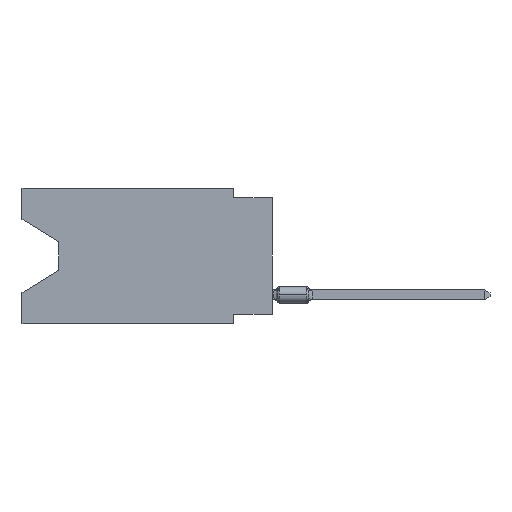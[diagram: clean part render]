
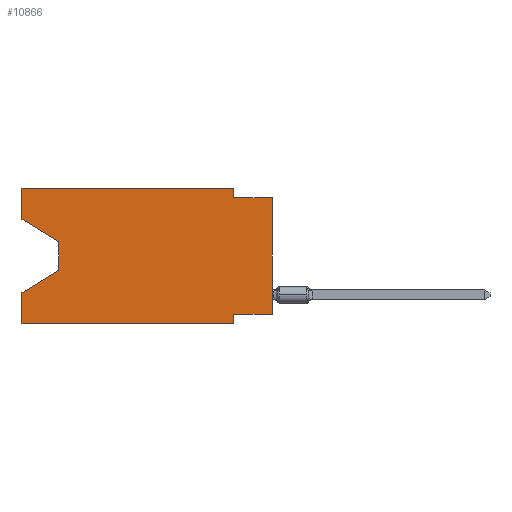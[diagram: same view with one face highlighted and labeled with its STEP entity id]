
A CAD part, left-side view. The second image highlights one B-rep face of the part: STEP entity #10866.
In plain terms, the highlighted planar face has unit normal (-1, 0, 0).
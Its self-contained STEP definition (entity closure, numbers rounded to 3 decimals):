
#94 = CARTESIAN_POINT ( 'NONE',  ( 0., 16.383, -2.038 ) ) ;
#161 = CARTESIAN_POINT ( 'NONE',  ( 0., 16.383, -6.852 ) ) ;
#174 = EDGE_CURVE ( 'NONE', #10808, #25910, #8458, .T. ) ;
#199 = CARTESIAN_POINT ( 'NONE',  ( 0., 16.383, 0. ) ) ;
#316 = DIRECTION ( 'NONE',  ( 0., 0., 1. ) ) ;
#1259 = ORIENTED_EDGE ( 'NONE', *, *, #18233, .T. ) ;
#1653 = VERTEX_POINT ( 'NONE', #4019 ) ;
#1872 = VECTOR ( 'NONE', #27531, 1000. ) ;
#2464 = CARTESIAN_POINT ( 'NONE',  ( 0., 2.54, -8.89 ) ) ;
#2564 = LINE ( 'NONE', #18908, #8574 ) ;
#3318 = VERTEX_POINT ( 'NONE', #94 ) ;
#3517 = LINE ( 'NONE', #28658, #28366 ) ;
#3856 = VECTOR ( 'NONE', #316, 1000. ) ;
#4019 = CARTESIAN_POINT ( 'NONE',  ( 0., 0., -0.635 ) ) ;
#4027 = CARTESIAN_POINT ( 'NONE',  ( 0., 13.97, -3.505 ) ) ;
#4533 = VECTOR ( 'NONE', #28274, 1000. ) ;
#4582 = CARTESIAN_POINT ( 'NONE',  ( 0., 2.54, 0. ) ) ;
#4903 = CARTESIAN_POINT ( 'NONE',  ( 0., 16.383, -2.038 ) ) ;
#4917 = ORIENTED_EDGE ( 'NONE', *, *, #6311, .T. ) ;
#5042 = CARTESIAN_POINT ( 'NONE',  ( 0., 13.97, -3.505 ) ) ;
#5176 = CARTESIAN_POINT ( 'NONE',  ( 0., 0., 0. ) ) ;
#5180 = VECTOR ( 'NONE', #23987, 1000. ) ;
#6311 = EDGE_CURVE ( 'NONE', #16733, #1653, #12278, .T. ) ;
#6521 = EDGE_CURVE ( 'NONE', #3318, #10808, #12084, .T. ) ;
#8110 = CARTESIAN_POINT ( 'NONE',  ( 0., 16.383, -8.89 ) ) ;
#8245 = ORIENTED_EDGE ( 'NONE', *, *, #27489, .F. ) ;
#8458 = LINE ( 'NONE', #24808, #15820 ) ;
#8574 = VECTOR ( 'NONE', #14290, 1000. ) ;
#9276 = CARTESIAN_POINT ( 'NONE',  ( 0., 16.383, 0. ) ) ;
#9345 = LINE ( 'NONE', #23687, #5180 ) ;
#9678 = ORIENTED_EDGE ( 'NONE', *, *, #19891, .T. ) ;
#9737 = VECTOR ( 'NONE', #12113, 1000. ) ;
#10376 = CARTESIAN_POINT ( 'NONE',  ( 0., 2.54, -0.635 ) ) ;
#10411 = LINE ( 'NONE', #19818, #9737 ) ;
#10499 = ORIENTED_EDGE ( 'NONE', *, *, #20463, .T. ) ;
#10564 = EDGE_CURVE ( 'NONE', #14357, #25654, #2564, .T. ) ;
#10687 = ORIENTED_EDGE ( 'NONE', *, *, #10564, .F. ) ;
#10729 = VERTEX_POINT ( 'NONE', #8110 ) ;
#10808 = VERTEX_POINT ( 'NONE', #13043 ) ;
#10866 = ADVANCED_FACE ( 'NONE', ( #27672 ), #20418, .F. ) ;
#11349 = VERTEX_POINT ( 'NONE', #161 ) ;
#11855 = CARTESIAN_POINT ( 'NONE',  ( 0., 2.54, -8.255 ) ) ;
#11998 = DIRECTION ( 'NONE',  ( 0., -0.855, -0.519 ) ) ;
#12084 = LINE ( 'NONE', #199, #4533 ) ;
#12113 = DIRECTION ( 'NONE',  ( 0., 0.855, -0.519 ) ) ;
#12263 = VERTEX_POINT ( 'NONE', #20882 ) ;
#12278 = LINE ( 'NONE', #5176, #25726 ) ;
#13043 = CARTESIAN_POINT ( 'NONE',  ( 0., 16.383, 0. ) ) ;
#13318 = ORIENTED_EDGE ( 'NONE', *, *, #24671, .F. ) ;
#13507 = LINE ( 'NONE', #15665, #22128 ) ;
#13980 = EDGE_CURVE ( 'NONE', #10729, #11349, #28088, .T. ) ;
#14290 = DIRECTION ( 'NONE',  ( 0., 0., -1. ) ) ;
#14357 = VERTEX_POINT ( 'NONE', #11855 ) ;
#14587 = DIRECTION ( 'NONE',  ( 0., 0., 1. ) ) ;
#15665 = CARTESIAN_POINT ( 'NONE',  ( 0., 0., -0.635 ) ) ;
#15820 = VECTOR ( 'NONE', #18325, 1000. ) ;
#16733 = VERTEX_POINT ( 'NONE', #27047 ) ;
#18233 = EDGE_CURVE ( 'NONE', #30322, #12263, #25317, .T. ) ;
#18325 = DIRECTION ( 'NONE',  ( 0., -1., 0. ) ) ;
#18405 = EDGE_LOOP ( 'NONE', ( #9678, #1259, #10499, #20678, #25299, #10687, #13318, #4917, #8245, #21248, #18439, #27879 ) ) ;
#18439 = ORIENTED_EDGE ( 'NONE', *, *, #174, .F. ) ;
#18583 = VECTOR ( 'NONE', #11998, 1000. ) ;
#18908 = CARTESIAN_POINT ( 'NONE',  ( 0., 2.54, -8.89 ) ) ;
#19818 = CARTESIAN_POINT ( 'NONE',  ( 0., 13.97, -5.385 ) ) ;
#19891 = EDGE_CURVE ( 'NONE', #3318, #30322, #30501, .T. ) ;
#20418 = PLANE ( 'NONE',  #20900 ) ;
#20463 = EDGE_CURVE ( 'NONE', #12263, #11349, #10411, .T. ) ;
#20676 = DIRECTION ( 'NONE',  ( 0., 0., -1. ) ) ;
#20678 = ORIENTED_EDGE ( 'NONE', *, *, #13980, .F. ) ;
#20882 = CARTESIAN_POINT ( 'NONE',  ( 0., 13.97, -5.385 ) ) ;
#20900 = AXIS2_PLACEMENT_3D ( 'NONE', #27524, #29981, #27366 ) ;
#21248 = ORIENTED_EDGE ( 'NONE', *, *, #22199, .F. ) ;
#21576 = VERTEX_POINT ( 'NONE', #10376 ) ;
#22128 = VECTOR ( 'NONE', #27380, 1000. ) ;
#22199 = EDGE_CURVE ( 'NONE', #25910, #21576, #9345, .T. ) ;
#23687 = CARTESIAN_POINT ( 'NONE',  ( 0., 2.54, 0. ) ) ;
#23987 = DIRECTION ( 'NONE',  ( 0., 0., -1. ) ) ;
#24671 = EDGE_CURVE ( 'NONE', #16733, #14357, #3517, .T. ) ;
#24808 = CARTESIAN_POINT ( 'NONE',  ( 0., 16.383, 0. ) ) ;
#24916 = LINE ( 'NONE', #29529, #1872 ) ;
#25299 = ORIENTED_EDGE ( 'NONE', *, *, #28884, .T. ) ;
#25317 = LINE ( 'NONE', #4027, #26411 ) ;
#25654 = VERTEX_POINT ( 'NONE', #2464 ) ;
#25726 = VECTOR ( 'NONE', #14587, 1000. ) ;
#25910 = VERTEX_POINT ( 'NONE', #4582 ) ;
#26411 = VECTOR ( 'NONE', #20676, 1000. ) ;
#26814 = DIRECTION ( 'NONE',  ( 0., 1., 0. ) ) ;
#27047 = CARTESIAN_POINT ( 'NONE',  ( 0., 0., -8.255 ) ) ;
#27366 = DIRECTION ( 'NONE',  ( 0., 0., -1. ) ) ;
#27380 = DIRECTION ( 'NONE',  ( 0., -1., 0. ) ) ;
#27489 = EDGE_CURVE ( 'NONE', #21576, #1653, #13507, .T. ) ;
#27524 = CARTESIAN_POINT ( 'NONE',  ( 0., 16.383, 0. ) ) ;
#27531 = DIRECTION ( 'NONE',  ( 0., -1., 0. ) ) ;
#27672 = FACE_OUTER_BOUND ( 'NONE', #18405, .T. ) ;
#27879 = ORIENTED_EDGE ( 'NONE', *, *, #6521, .F. ) ;
#28088 = LINE ( 'NONE', #9276, #3856 ) ;
#28274 = DIRECTION ( 'NONE',  ( 0., 0., 1. ) ) ;
#28366 = VECTOR ( 'NONE', #26814, 1000. ) ;
#28658 = CARTESIAN_POINT ( 'NONE',  ( 0., 0., -8.255 ) ) ;
#28884 = EDGE_CURVE ( 'NONE', #10729, #25654, #24916, .T. ) ;
#29529 = CARTESIAN_POINT ( 'NONE',  ( 0., 16.383, -8.89 ) ) ;
#29981 = DIRECTION ( 'NONE',  ( 1., 0., 0. ) ) ;
#30322 = VERTEX_POINT ( 'NONE', #5042 ) ;
#30501 = LINE ( 'NONE', #4903, #18583 ) ;
